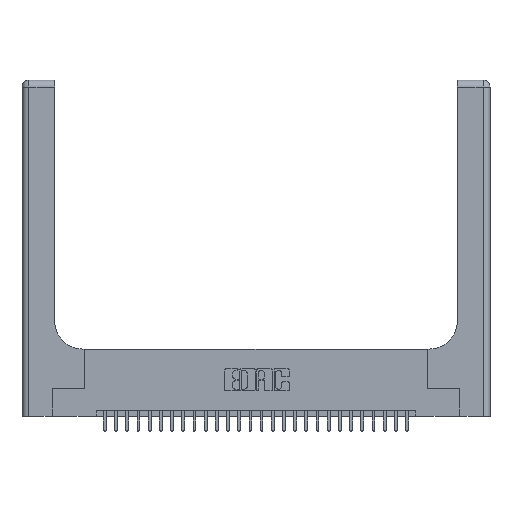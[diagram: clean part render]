
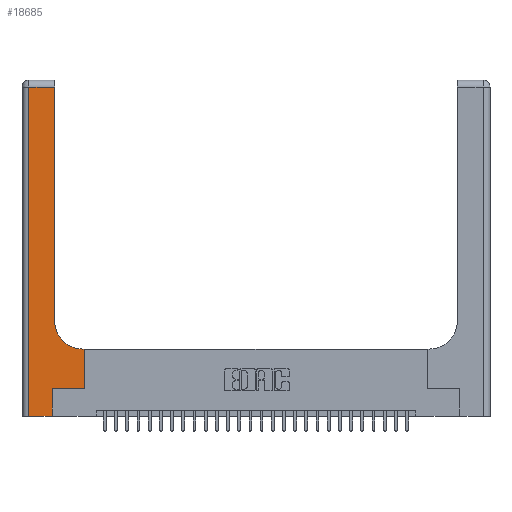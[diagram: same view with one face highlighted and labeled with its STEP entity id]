
A CAD part, top view. The second image highlights one B-rep face of the part: STEP entity #18685.
In plain terms, the highlighted planar face has unit normal (0, 0, 1).
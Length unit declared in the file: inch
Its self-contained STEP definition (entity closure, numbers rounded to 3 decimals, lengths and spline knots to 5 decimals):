
#170 = VERTEX_POINT ( 'NONE', #9626 ) ;
#354 = CARTESIAN_POINT ( 'NONE',  ( 0.06, 3., 0.37 ) ) ;
#777 = CARTESIAN_POINT ( 'NONE',  ( 0., 3., 0.37 ) ) ;
#1024 = LINE ( 'NONE', #6316, #21044 ) ;
#1994 = VERTEX_POINT ( 'NONE', #4713 ) ;
#2723 = VECTOR ( 'NONE', #19601, 39.37008 ) ;
#3024 = EDGE_CURVE ( 'NONE', #1994, #8233, #11829, .T. ) ;
#3033 = DIRECTION ( 'NONE',  ( 0., 0., -1. ) ) ;
#4416 = LINE ( 'NONE', #354, #14193 ) ;
#4713 = CARTESIAN_POINT ( 'NONE',  ( 0.5585, 0.6, 0.37 ) ) ;
#5028 = LINE ( 'NONE', #25648, #23343 ) ;
#6005 = DIRECTION ( 'NONE',  ( 0., 1., 0. ) ) ;
#6316 = CARTESIAN_POINT ( 'NONE',  ( 0.5585, 0.25, 0.37 ) ) ;
#6498 = CARTESIAN_POINT ( 'NONE',  ( 0.5415, 0.85, 0.37 ) ) ;
#6898 = DIRECTION ( 'NONE',  ( 1., 0., 0. ) ) ;
#7245 = ORIENTED_EDGE ( 'NONE', *, *, #26686, .T. ) ;
#7460 = VECTOR ( 'NONE', #6898, 39.37008 ) ;
#8233 = VERTEX_POINT ( 'NONE', #12909 ) ;
#9060 = FACE_OUTER_BOUND ( 'NONE', #17806, .T. ) ;
#9081 = DIRECTION ( 'NONE',  ( 0., -1., 0. ) ) ;
#9626 = CARTESIAN_POINT ( 'NONE',  ( 0.06, 0., 0.37 ) ) ;
#10004 = LINE ( 'NONE', #24647, #12105 ) ;
#10105 = PLANE ( 'NONE',  #19928 ) ;
#10668 = AXIS2_PLACEMENT_3D ( 'NONE', #6498, #17593, #19940 ) ;
#10698 = VERTEX_POINT ( 'NONE', #27392 ) ;
#10829 = CARTESIAN_POINT ( 'NONE',  ( 0.2915, 0.85, 0.37 ) ) ;
#11829 = LINE ( 'NONE', #19392, #2723 ) ;
#12105 = VECTOR ( 'NONE', #28978, 39.37008 ) ;
#12909 = CARTESIAN_POINT ( 'NONE',  ( 0.5415, 0.6, 0.37 ) ) ;
#13174 = ORIENTED_EDGE ( 'NONE', *, *, #28254, .T. ) ;
#13546 = VERTEX_POINT ( 'NONE', #24408 ) ;
#14193 = VECTOR ( 'NONE', #9081, 39.37008 ) ;
#14594 = LINE ( 'NONE', #26571, #18462 ) ;
#14878 = EDGE_CURVE ( 'NONE', #10698, #24489, #18018, .T. ) ;
#15215 = VERTEX_POINT ( 'NONE', #10829 ) ;
#15321 = DIRECTION ( 'NONE',  ( 0., 1., 0. ) ) ;
#15788 = EDGE_CURVE ( 'NONE', #8233, #15215, #16914, .T. ) ;
#16125 = VERTEX_POINT ( 'NONE', #22858 ) ;
#16914 = CIRCLE ( 'NONE', #10668, 0.25 ) ;
#17593 = DIRECTION ( 'NONE',  ( 0., 0., -1. ) ) ;
#17806 = EDGE_LOOP ( 'NONE', ( #24353, #23968, #26988, #7245, #13174, #21404, #23685, #19657, #18192 ) ) ;
#17841 = DIRECTION ( 'NONE',  ( 0., 1., 0. ) ) ;
#17861 = VECTOR ( 'NONE', #17841, 39.37008 ) ;
#18018 = LINE ( 'NONE', #27269, #7460 ) ;
#18192 = ORIENTED_EDGE ( 'NONE', *, *, #15788, .T. ) ;
#18462 = VECTOR ( 'NONE', #6005, 39.37008 ) ;
#18652 = DIRECTION ( 'NONE',  ( 1., 0., 0. ) ) ;
#18685 = ADVANCED_FACE ( 'NONE', ( #9060 ), #10105, .F. ) ;
#19392 = CARTESIAN_POINT ( 'NONE',  ( 0.2915, 0.6, 0.37 ) ) ;
#19601 = DIRECTION ( 'NONE',  ( -1., 0., 0. ) ) ;
#19657 = ORIENTED_EDGE ( 'NONE', *, *, #3024, .T. ) ;
#19928 = AXIS2_PLACEMENT_3D ( 'NONE', #777, #3033, #21297 ) ;
#19940 = DIRECTION ( 'NONE',  ( 1., 0., 0. ) ) ;
#19950 = EDGE_CURVE ( 'NONE', #15215, #21604, #14594, .T. ) ;
#20667 = LINE ( 'NONE', #26818, #17861 ) ;
#20763 = EDGE_CURVE ( 'NONE', #21604, #16125, #10004, .T. ) ;
#21044 = VECTOR ( 'NONE', #15321, 39.37008 ) ;
#21297 = DIRECTION ( 'NONE',  ( -1., 0., 0. ) ) ;
#21404 = ORIENTED_EDGE ( 'NONE', *, *, #14878, .T. ) ;
#21604 = VERTEX_POINT ( 'NONE', #26185 ) ;
#22858 = CARTESIAN_POINT ( 'NONE',  ( 0.06, 2.94, 0.37 ) ) ;
#23343 = VECTOR ( 'NONE', #18652, 39.37008 ) ;
#23628 = CARTESIAN_POINT ( 'NONE',  ( 0.5585, 0.25, 0.37 ) ) ;
#23685 = ORIENTED_EDGE ( 'NONE', *, *, #23950, .T. ) ;
#23950 = EDGE_CURVE ( 'NONE', #24489, #1994, #1024, .T. ) ;
#23968 = ORIENTED_EDGE ( 'NONE', *, *, #20763, .T. ) ;
#24353 = ORIENTED_EDGE ( 'NONE', *, *, #19950, .T. ) ;
#24408 = CARTESIAN_POINT ( 'NONE',  ( 0.269, 0., 0.37 ) ) ;
#24489 = VERTEX_POINT ( 'NONE', #23628 ) ;
#24647 = CARTESIAN_POINT ( 'NONE',  ( 0., 2.94, 0.37 ) ) ;
#25648 = CARTESIAN_POINT ( 'NONE',  ( 0., 0., 0.37 ) ) ;
#25896 = EDGE_CURVE ( 'NONE', #16125, #170, #4416, .T. ) ;
#26185 = CARTESIAN_POINT ( 'NONE',  ( 0.2915, 2.94, 0.37 ) ) ;
#26571 = CARTESIAN_POINT ( 'NONE',  ( 0.2915, 3., 0.37 ) ) ;
#26686 = EDGE_CURVE ( 'NONE', #170, #13546, #5028, .T. ) ;
#26818 = CARTESIAN_POINT ( 'NONE',  ( 0.269, 0., 0.37 ) ) ;
#26988 = ORIENTED_EDGE ( 'NONE', *, *, #25896, .T. ) ;
#27269 = CARTESIAN_POINT ( 'NONE',  ( 0.269, 0.25, 0.37 ) ) ;
#27392 = CARTESIAN_POINT ( 'NONE',  ( 0.269, 0.25, 0.37 ) ) ;
#28254 = EDGE_CURVE ( 'NONE', #13546, #10698, #20667, .T. ) ;
#28978 = DIRECTION ( 'NONE',  ( -1., 0., 0. ) ) ;
